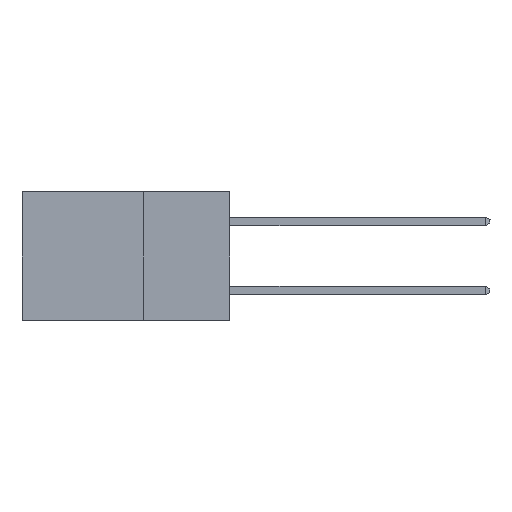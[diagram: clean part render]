
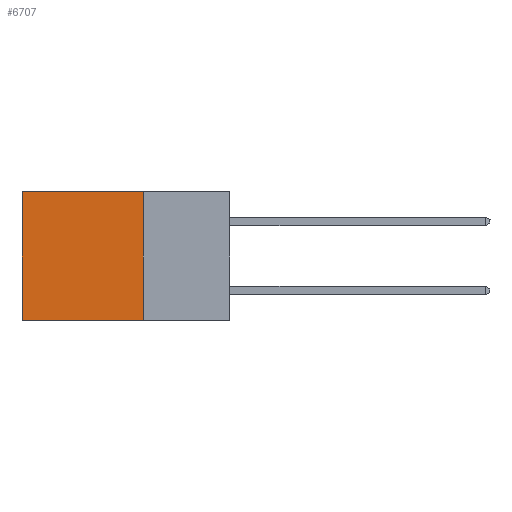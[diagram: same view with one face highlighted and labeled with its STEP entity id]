
A CAD part, left-side view. The second image highlights one B-rep face of the part: STEP entity #6707.
In plain terms, the highlighted planar face has unit normal (-1, 0, 0).
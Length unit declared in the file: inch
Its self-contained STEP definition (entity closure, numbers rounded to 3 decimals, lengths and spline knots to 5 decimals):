
#414 = VECTOR ( 'NONE', #3122, 39.37008 ) ;
#573 = ORIENTED_EDGE ( 'NONE', *, *, #8280, .F. ) ;
#1016 = CARTESIAN_POINT ( 'NONE',  ( 0.2615, 0.25, -0.37 ) ) ;
#1091 = CARTESIAN_POINT ( 'NONE',  ( 0.2615, 0.25, -0.37 ) ) ;
#2748 = CARTESIAN_POINT ( 'NONE',  ( 0.2615, 0.25, 0. ) ) ;
#3122 = DIRECTION ( 'NONE',  ( 0., 0., -1. ) ) ;
#3269 = CARTESIAN_POINT ( 'NONE',  ( 0.2615, 0.6, -0.37 ) ) ;
#3669 = VERTEX_POINT ( 'NONE', #6615 ) ;
#3999 = LINE ( 'NONE', #6711, #6942 ) ;
#4310 = DIRECTION ( 'NONE',  ( 0., 0., -1. ) ) ;
#4412 = EDGE_LOOP ( 'NONE', ( #9347, #14566, #573, #5911 ) ) ;
#4693 = VERTEX_POINT ( 'NONE', #5056 ) ;
#5056 = CARTESIAN_POINT ( 'NONE',  ( 0.2615, 0.6, -0.37 ) ) ;
#5454 = EDGE_CURVE ( 'NONE', #7300, #4693, #5640, .T. ) ;
#5589 = AXIS2_PLACEMENT_3D ( 'NONE', #1091, #12975, #5794 ) ;
#5640 = LINE ( 'NONE', #1016, #14889 ) ;
#5641 = FACE_OUTER_BOUND ( 'NONE', #4412, .T. ) ;
#5794 = DIRECTION ( 'NONE',  ( 0., 0., -1. ) ) ;
#5911 = ORIENTED_EDGE ( 'NONE', *, *, #7547, .T. ) ;
#6615 = CARTESIAN_POINT ( 'NONE',  ( 0.2615, 0.6, 0. ) ) ;
#6707 = ADVANCED_FACE ( 'NONE', ( #5641 ), #11594, .F. ) ;
#6711 = CARTESIAN_POINT ( 'NONE',  ( 0.2615, 0.25, -0.37 ) ) ;
#6925 = LINE ( 'NONE', #10688, #13274 ) ;
#6942 = VECTOR ( 'NONE', #4310, 39.37008 ) ;
#7300 = VERTEX_POINT ( 'NONE', #14089 ) ;
#7363 = VERTEX_POINT ( 'NONE', #2748 ) ;
#7547 = EDGE_CURVE ( 'NONE', #7363, #3669, #6925, .T. ) ;
#7918 = LINE ( 'NONE', #3269, #414 ) ;
#7966 = DIRECTION ( 'NONE',  ( 0., 1., 0. ) ) ;
#8280 = EDGE_CURVE ( 'NONE', #7363, #7300, #3999, .T. ) ;
#9347 = ORIENTED_EDGE ( 'NONE', *, *, #14680, .T. ) ;
#10688 = CARTESIAN_POINT ( 'NONE',  ( 0.2615, 0.25, 0. ) ) ;
#11594 = PLANE ( 'NONE',  #5589 ) ;
#12627 = DIRECTION ( 'NONE',  ( 0., 1., 0. ) ) ;
#12975 = DIRECTION ( 'NONE',  ( 1., 0., 0. ) ) ;
#13274 = VECTOR ( 'NONE', #12627, 39.37008 ) ;
#14089 = CARTESIAN_POINT ( 'NONE',  ( 0.2615, 0.25, -0.37 ) ) ;
#14566 = ORIENTED_EDGE ( 'NONE', *, *, #5454, .F. ) ;
#14680 = EDGE_CURVE ( 'NONE', #3669, #4693, #7918, .T. ) ;
#14889 = VECTOR ( 'NONE', #7966, 39.37008 ) ;
